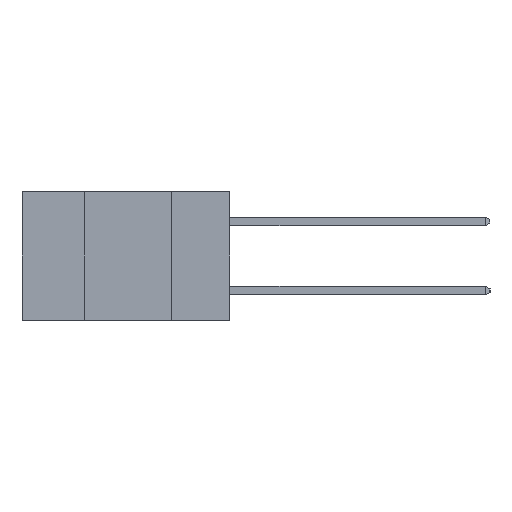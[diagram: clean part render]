
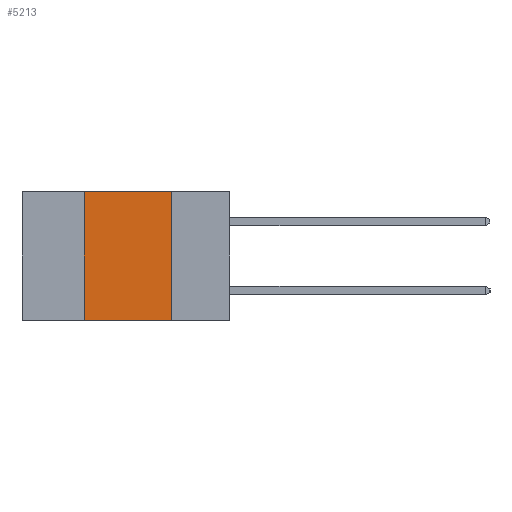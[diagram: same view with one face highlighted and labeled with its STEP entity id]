
A CAD part, left-side view. The second image highlights one B-rep face of the part: STEP entity #5213.
In plain terms, the highlighted planar face has unit normal (-1, 0, 0).
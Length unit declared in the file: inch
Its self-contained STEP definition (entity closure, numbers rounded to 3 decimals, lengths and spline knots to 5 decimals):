
#3861 = LINE ( 'NONE', #21267, #9938 ) ;
#5213 = ADVANCED_FACE ( 'NONE', ( #9876 ), #21102, .F. ) ;
#5789 = EDGE_CURVE ( 'NONE', #11156, #12800, #11484, .T. ) ;
#6669 = CARTESIAN_POINT ( 'NONE',  ( 0., 0.17, -0.37 ) ) ;
#7911 = ORIENTED_EDGE ( 'NONE', *, *, #19025, .F. ) ;
#8005 = EDGE_LOOP ( 'NONE', ( #24842, #7911, #11832, #16871 ) ) ;
#8324 = LINE ( 'NONE', #17407, #23728 ) ;
#8997 = CARTESIAN_POINT ( 'NONE',  ( 0., 0.6, 0. ) ) ;
#9146 = DIRECTION ( 'NONE',  ( 0., 0., 1. ) ) ;
#9202 = VERTEX_POINT ( 'NONE', #13683 ) ;
#9876 = FACE_OUTER_BOUND ( 'NONE', #8005, .T. ) ;
#9938 = VECTOR ( 'NONE', #9146, 39.37008 ) ;
#10717 = CARTESIAN_POINT ( 'NONE',  ( 0., 0.17, 0. ) ) ;
#11122 = DIRECTION ( 'NONE',  ( 0., 0., -1. ) ) ;
#11156 = VERTEX_POINT ( 'NONE', #10717 ) ;
#11484 = LINE ( 'NONE', #6669, #16843 ) ;
#11586 = VECTOR ( 'NONE', #18319, 39.37008 ) ;
#11832 = ORIENTED_EDGE ( 'NONE', *, *, #23961, .F. ) ;
#12643 = CARTESIAN_POINT ( 'NONE',  ( 0., 0.17, -0.37 ) ) ;
#12800 = VERTEX_POINT ( 'NONE', #12643 ) ;
#13683 = CARTESIAN_POINT ( 'NONE',  ( 0., 0.42, -0.37 ) ) ;
#14312 = CARTESIAN_POINT ( 'NONE',  ( 0., 0.6, -0.37 ) ) ;
#16751 = DIRECTION ( 'NONE',  ( 0., 0., -1. ) ) ;
#16843 = VECTOR ( 'NONE', #16751, 39.37008 ) ;
#16871 = ORIENTED_EDGE ( 'NONE', *, *, #20033, .T. ) ;
#16941 = LINE ( 'NONE', #14312, #11586 ) ;
#17407 = CARTESIAN_POINT ( 'NONE',  ( 0., 0.6, 0. ) ) ;
#18319 = DIRECTION ( 'NONE',  ( 0., -1., 0. ) ) ;
#19025 = EDGE_CURVE ( 'NONE', #23618, #11156, #8324, .T. ) ;
#19402 = DIRECTION ( 'NONE',  ( 0., -1., 0. ) ) ;
#20033 = EDGE_CURVE ( 'NONE', #9202, #12800, #16941, .T. ) ;
#21102 = PLANE ( 'NONE',  #25336 ) ;
#21267 = CARTESIAN_POINT ( 'NONE',  ( 0., 0.42, -0.37 ) ) ;
#22287 = CARTESIAN_POINT ( 'NONE',  ( 0., 0.42, 0. ) ) ;
#23058 = DIRECTION ( 'NONE',  ( 1., 0., 0. ) ) ;
#23618 = VERTEX_POINT ( 'NONE', #22287 ) ;
#23728 = VECTOR ( 'NONE', #19402, 39.37008 ) ;
#23961 = EDGE_CURVE ( 'NONE', #9202, #23618, #3861, .T. ) ;
#24842 = ORIENTED_EDGE ( 'NONE', *, *, #5789, .F. ) ;
#25336 = AXIS2_PLACEMENT_3D ( 'NONE', #8997, #23058, #11122 ) ;
